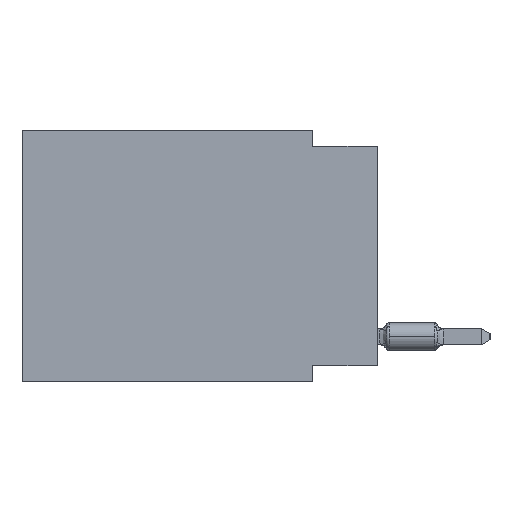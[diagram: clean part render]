
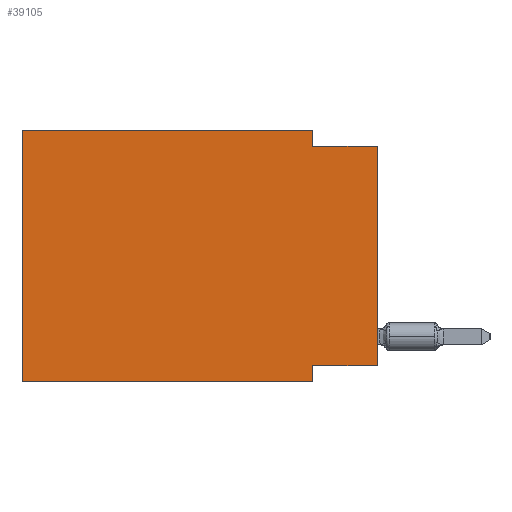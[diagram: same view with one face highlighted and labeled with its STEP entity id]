
A CAD part, left-side view. The second image highlights one B-rep face of the part: STEP entity #39105.
In plain terms, the highlighted planar face has unit normal (-1, 0, 0).
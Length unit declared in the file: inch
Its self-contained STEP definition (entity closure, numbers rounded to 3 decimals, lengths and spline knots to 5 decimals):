
#730 = ORIENTED_EDGE ( 'NONE', *, *, #3453, .F. ) ;
#924 = VECTOR ( 'NONE', #27955, 39.37008 ) ;
#1038 = CARTESIAN_POINT ( 'NONE',  ( 0., 0.1, 0. ) ) ;
#1401 = VECTOR ( 'NONE', #8125, 39.37008 ) ;
#1732 = ORIENTED_EDGE ( 'NONE', *, *, #13100, .T. ) ;
#1760 = CARTESIAN_POINT ( 'NONE',  ( 0., 0.55, 0. ) ) ;
#2477 = VERTEX_POINT ( 'NONE', #35111 ) ;
#3342 = EDGE_CURVE ( 'NONE', #27228, #18375, #38377, .T. ) ;
#3453 = EDGE_CURVE ( 'NONE', #20915, #2477, #30036, .T. ) ;
#5766 = VECTOR ( 'NONE', #37172, 39.37008 ) ;
#6384 = ORIENTED_EDGE ( 'NONE', *, *, #3342, .F. ) ;
#6780 = DIRECTION ( 'NONE',  ( 0., -1., 0. ) ) ;
#7564 = EDGE_CURVE ( 'NONE', #2477, #15002, #32667, .T. ) ;
#7699 = VECTOR ( 'NONE', #27364, 39.37008 ) ;
#8125 = DIRECTION ( 'NONE',  ( 0., -1., 0. ) ) ;
#8733 = VERTEX_POINT ( 'NONE', #29426 ) ;
#9482 = LINE ( 'NONE', #9717, #924 ) ;
#9516 = CARTESIAN_POINT ( 'NONE',  ( 0., 0.1, -0.39 ) ) ;
#9717 = CARTESIAN_POINT ( 'NONE',  ( 0., 0., -0.025 ) ) ;
#10867 = EDGE_LOOP ( 'NONE', ( #19520, #28326, #22642, #730, #21620, #1732, #18787, #6384 ) ) ;
#11602 = AXIS2_PLACEMENT_3D ( 'NONE', #1760, #43570, #15830 ) ;
#12214 = EDGE_CURVE ( 'NONE', #15002, #39677, #9482, .T. ) ;
#13100 = EDGE_CURVE ( 'NONE', #8733, #16394, #41877, .T. ) ;
#14587 = DIRECTION ( 'NONE',  ( 0., 1., 0. ) ) ;
#14666 = LINE ( 'NONE', #36380, #32400 ) ;
#15002 = VERTEX_POINT ( 'NONE', #18340 ) ;
#15478 = VECTOR ( 'NONE', #19463, 39.37008 ) ;
#15830 = DIRECTION ( 'NONE',  ( 0., 0., -1. ) ) ;
#16027 = DIRECTION ( 'NONE',  ( 0., 0., -1. ) ) ;
#16394 = VERTEX_POINT ( 'NONE', #9516 ) ;
#17697 = VECTOR ( 'NONE', #14587, 39.37008 ) ;
#18063 = CARTESIAN_POINT ( 'NONE',  ( 0., 0.1, -0.365 ) ) ;
#18340 = CARTESIAN_POINT ( 'NONE',  ( 0., 0.1, -0.025 ) ) ;
#18375 = VERTEX_POINT ( 'NONE', #18063 ) ;
#18787 = ORIENTED_EDGE ( 'NONE', *, *, #43398, .F. ) ;
#19463 = DIRECTION ( 'NONE',  ( 0., 0., -1. ) ) ;
#19520 = ORIENTED_EDGE ( 'NONE', *, *, #40104, .T. ) ;
#20915 = VERTEX_POINT ( 'NONE', #39481 ) ;
#21184 = VECTOR ( 'NONE', #6780, 39.37008 ) ;
#21620 = ORIENTED_EDGE ( 'NONE', *, *, #30762, .F. ) ;
#22642 = ORIENTED_EDGE ( 'NONE', *, *, #7564, .F. ) ;
#23088 = CARTESIAN_POINT ( 'NONE',  ( 0., 0., 0. ) ) ;
#26026 = FACE_OUTER_BOUND ( 'NONE', #10867, .T. ) ;
#26771 = CARTESIAN_POINT ( 'NONE',  ( 0., 0., -0.365 ) ) ;
#27228 = VERTEX_POINT ( 'NONE', #26771 ) ;
#27364 = DIRECTION ( 'NONE',  ( 0., 0., 1. ) ) ;
#27473 = LINE ( 'NONE', #23088, #5766 ) ;
#27955 = DIRECTION ( 'NONE',  ( 0., -1., 0. ) ) ;
#28326 = ORIENTED_EDGE ( 'NONE', *, *, #12214, .F. ) ;
#29426 = CARTESIAN_POINT ( 'NONE',  ( 0., 0.55, -0.39 ) ) ;
#30036 = LINE ( 'NONE', #44131, #1401 ) ;
#30762 = EDGE_CURVE ( 'NONE', #8733, #20915, #44905, .T. ) ;
#32400 = VECTOR ( 'NONE', #16027, 39.37008 ) ;
#32667 = LINE ( 'NONE', #1038, #15478 ) ;
#35111 = CARTESIAN_POINT ( 'NONE',  ( 0., 0.1, 0. ) ) ;
#36380 = CARTESIAN_POINT ( 'NONE',  ( 0., 0.1, -0.39 ) ) ;
#37172 = DIRECTION ( 'NONE',  ( 0., 0., 1. ) ) ;
#38377 = LINE ( 'NONE', #43016, #17697 ) ;
#38402 = CARTESIAN_POINT ( 'NONE',  ( 0., 0.55, -0.39 ) ) ;
#38417 = CARTESIAN_POINT ( 'NONE',  ( 0., 0.55, 0. ) ) ;
#39105 = ADVANCED_FACE ( 'NONE', ( #26026 ), #43795, .F. ) ;
#39481 = CARTESIAN_POINT ( 'NONE',  ( 0., 0.55, 0. ) ) ;
#39677 = VERTEX_POINT ( 'NONE', #41594 ) ;
#40104 = EDGE_CURVE ( 'NONE', #27228, #39677, #27473, .T. ) ;
#41594 = CARTESIAN_POINT ( 'NONE',  ( 0., 0., -0.025 ) ) ;
#41877 = LINE ( 'NONE', #38402, #21184 ) ;
#43016 = CARTESIAN_POINT ( 'NONE',  ( 0., 0., -0.365 ) ) ;
#43398 = EDGE_CURVE ( 'NONE', #18375, #16394, #14666, .T. ) ;
#43570 = DIRECTION ( 'NONE',  ( 1., 0., 0. ) ) ;
#43795 = PLANE ( 'NONE',  #11602 ) ;
#44131 = CARTESIAN_POINT ( 'NONE',  ( 0., 0.55, 0. ) ) ;
#44905 = LINE ( 'NONE', #38417, #7699 ) ;
